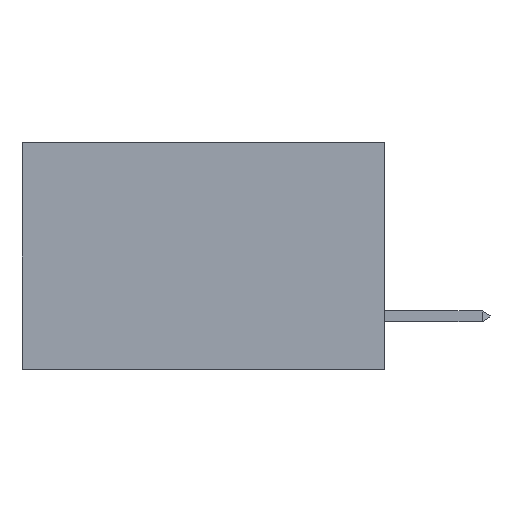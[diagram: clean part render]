
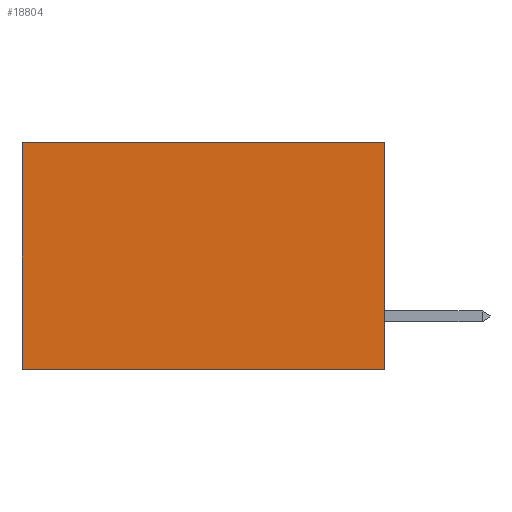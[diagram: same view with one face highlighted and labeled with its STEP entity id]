
A CAD part, left-side view. The second image highlights one B-rep face of the part: STEP entity #18804.
In plain terms, the highlighted planar face has unit normal (-1, 0, 0).
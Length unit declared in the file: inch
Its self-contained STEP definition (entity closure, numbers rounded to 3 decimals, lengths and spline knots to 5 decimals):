
#141 = CARTESIAN_POINT ( 'NONE',  ( 0.2875, 0., -0.375 ) ) ;
#265 = CARTESIAN_POINT ( 'NONE',  ( 0.2875, 0., -0.375 ) ) ;
#409 = DIRECTION ( 'NONE',  ( 0., 0., -1. ) ) ;
#457 = ORIENTED_EDGE ( 'NONE', *, *, #1981, .F. ) ;
#1946 = DIRECTION ( 'NONE',  ( 1., 0., 0. ) ) ;
#1981 = EDGE_CURVE ( 'NONE', #2110, #2902, #17196, .T. ) ;
#2110 = VERTEX_POINT ( 'NONE', #265 ) ;
#2271 = CARTESIAN_POINT ( 'NONE',  ( 0.2875, 0., -0.375 ) ) ;
#2902 = VERTEX_POINT ( 'NONE', #15550 ) ;
#3477 = ORIENTED_EDGE ( 'NONE', *, *, #7477, .T. ) ;
#3568 = LINE ( 'NONE', #11240, #20055 ) ;
#3636 = PLANE ( 'NONE',  #10348 ) ;
#4903 = CARTESIAN_POINT ( 'NONE',  ( 0.2875, 0., 0. ) ) ;
#7477 = EDGE_CURVE ( 'NONE', #8164, #2902, #19734, .T. ) ;
#8164 = VERTEX_POINT ( 'NONE', #14043 ) ;
#9503 = DIRECTION ( 'NONE',  ( 0., 1., 0. ) ) ;
#9706 = EDGE_CURVE ( 'NONE', #10029, #2110, #12721, .T. ) ;
#10029 = VERTEX_POINT ( 'NONE', #4903 ) ;
#10090 = EDGE_LOOP ( 'NONE', ( #3477, #457, #16356, #13673 ) ) ;
#10348 = AXIS2_PLACEMENT_3D ( 'NONE', #14602, #1946, #409 ) ;
#10811 = DIRECTION ( 'NONE',  ( 0., 0., -1. ) ) ;
#11240 = CARTESIAN_POINT ( 'NONE',  ( 0.2875, 0., 0. ) ) ;
#12464 = VECTOR ( 'NONE', #15050, 39.37008 ) ;
#12721 = LINE ( 'NONE', #2271, #12464 ) ;
#13673 = ORIENTED_EDGE ( 'NONE', *, *, #16808, .T. ) ;
#13997 = CARTESIAN_POINT ( 'NONE',  ( 0.2875, 0.6, -0.375 ) ) ;
#14043 = CARTESIAN_POINT ( 'NONE',  ( 0.2875, 0.6, 0. ) ) ;
#14602 = CARTESIAN_POINT ( 'NONE',  ( 0.2875, 0., -0.375 ) ) ;
#15050 = DIRECTION ( 'NONE',  ( 0., 0., -1. ) ) ;
#15238 = VECTOR ( 'NONE', #10811, 39.37008 ) ;
#15460 = VECTOR ( 'NONE', #16058, 39.37008 ) ;
#15550 = CARTESIAN_POINT ( 'NONE',  ( 0.2875, 0.6, -0.375 ) ) ;
#16058 = DIRECTION ( 'NONE',  ( 0., 1., 0. ) ) ;
#16356 = ORIENTED_EDGE ( 'NONE', *, *, #9706, .F. ) ;
#16808 = EDGE_CURVE ( 'NONE', #10029, #8164, #3568, .T. ) ;
#16958 = FACE_OUTER_BOUND ( 'NONE', #10090, .T. ) ;
#17196 = LINE ( 'NONE', #141, #15460 ) ;
#18804 = ADVANCED_FACE ( 'NONE', ( #16958 ), #3636, .F. ) ;
#19734 = LINE ( 'NONE', #13997, #15238 ) ;
#20055 = VECTOR ( 'NONE', #9503, 39.37008 ) ;
